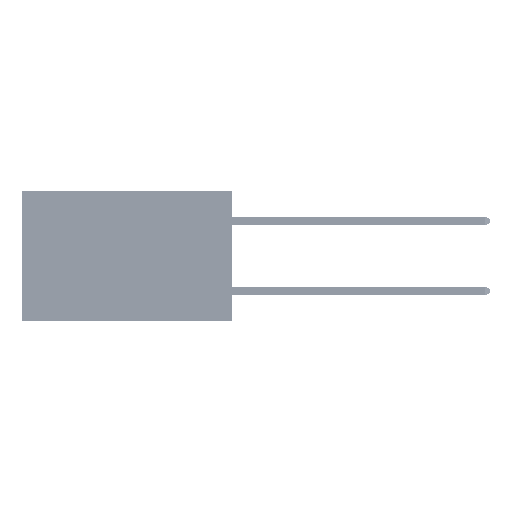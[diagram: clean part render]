
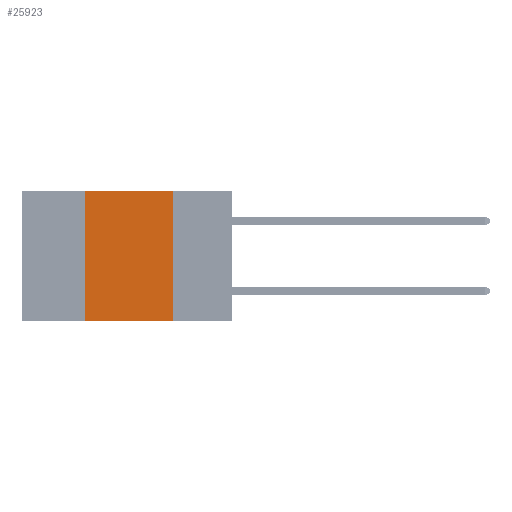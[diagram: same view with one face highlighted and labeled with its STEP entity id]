
A CAD part, left-side view. The second image highlights one B-rep face of the part: STEP entity #25923.
In plain terms, the highlighted planar face has unit normal (-1, 0, 0).
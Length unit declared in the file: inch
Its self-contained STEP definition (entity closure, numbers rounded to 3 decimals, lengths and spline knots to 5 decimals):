
#1164 = VERTEX_POINT ( 'NONE', #20975 ) ;
#2680 = EDGE_CURVE ( 'NONE', #45168, #1164, #38282, .T. ) ;
#6358 = DIRECTION ( 'NONE',  ( 0., 0., -1. ) ) ;
#7346 = DIRECTION ( 'NONE',  ( 1., 0., 0. ) ) ;
#9038 = VERTEX_POINT ( 'NONE', #33151 ) ;
#14002 = CARTESIAN_POINT ( 'NONE',  ( 0., 0.17, 0. ) ) ;
#15031 = ORIENTED_EDGE ( 'NONE', *, *, #34906, .F. ) ;
#15222 = PLANE ( 'NONE',  #32823 ) ;
#16908 = VECTOR ( 'NONE', #21056, 39.37008 ) ;
#17901 = VECTOR ( 'NONE', #6358, 39.37008 ) ;
#19346 = LINE ( 'NONE', #40112, #20150 ) ;
#19565 = VECTOR ( 'NONE', #49128, 39.37008 ) ;
#20150 = VECTOR ( 'NONE', #26714, 39.37008 ) ;
#20975 = CARTESIAN_POINT ( 'NONE',  ( 0., 0.17, -0.37 ) ) ;
#21056 = DIRECTION ( 'NONE',  ( 0., -1., 0. ) ) ;
#25923 = ADVANCED_FACE ( 'NONE', ( #30223 ), #15222, .F. ) ;
#26714 = DIRECTION ( 'NONE',  ( 0., 0., 1. ) ) ;
#26994 = VERTEX_POINT ( 'NONE', #47565 ) ;
#27848 = ORIENTED_EDGE ( 'NONE', *, *, #44908, .F. ) ;
#28741 = LINE ( 'NONE', #14002, #17901 ) ;
#30223 = FACE_OUTER_BOUND ( 'NONE', #30421, .T. ) ;
#30421 = EDGE_LOOP ( 'NONE', ( #34912, #15031, #27848, #32071 ) ) ;
#30727 = DIRECTION ( 'NONE',  ( 0., 0., -1. ) ) ;
#32071 = ORIENTED_EDGE ( 'NONE', *, *, #2680, .T. ) ;
#32736 = CARTESIAN_POINT ( 'NONE',  ( 0., 0.6, -0.37 ) ) ;
#32823 = AXIS2_PLACEMENT_3D ( 'NONE', #45508, #7346, #30727 ) ;
#33151 = CARTESIAN_POINT ( 'NONE',  ( 0., 0.42, 0. ) ) ;
#33459 = CARTESIAN_POINT ( 'NONE',  ( 0., 0.42, -0.37 ) ) ;
#34906 = EDGE_CURVE ( 'NONE', #9038, #26994, #41501, .T. ) ;
#34912 = ORIENTED_EDGE ( 'NONE', *, *, #49338, .F. ) ;
#38282 = LINE ( 'NONE', #32736, #16908 ) ;
#40112 = CARTESIAN_POINT ( 'NONE',  ( 0., 0.42, 0. ) ) ;
#41501 = LINE ( 'NONE', #48626, #19565 ) ;
#44908 = EDGE_CURVE ( 'NONE', #45168, #9038, #19346, .T. ) ;
#45168 = VERTEX_POINT ( 'NONE', #33459 ) ;
#45508 = CARTESIAN_POINT ( 'NONE',  ( 0., 0.6, 0. ) ) ;
#47565 = CARTESIAN_POINT ( 'NONE',  ( 0., 0.17, 0. ) ) ;
#48626 = CARTESIAN_POINT ( 'NONE',  ( 0., 0.6, 0. ) ) ;
#49128 = DIRECTION ( 'NONE',  ( 0., -1., 0. ) ) ;
#49338 = EDGE_CURVE ( 'NONE', #26994, #1164, #28741, .T. ) ;
